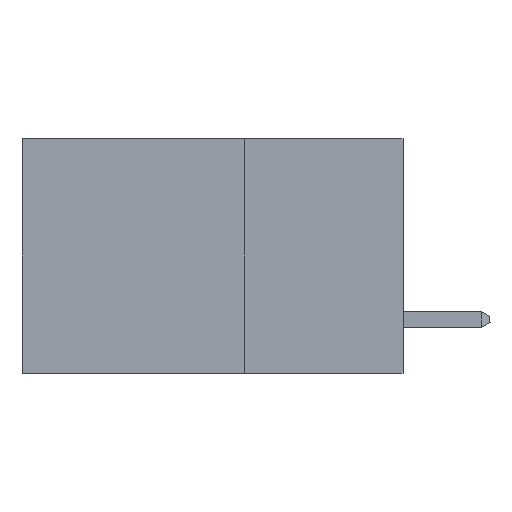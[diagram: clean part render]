
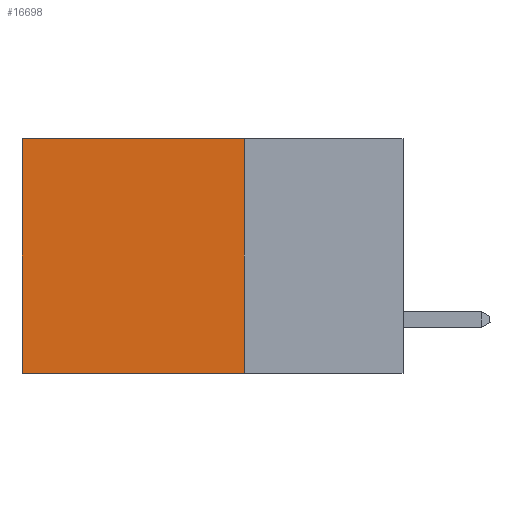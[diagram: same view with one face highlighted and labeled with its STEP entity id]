
A CAD part, left-side view. The second image highlights one B-rep face of the part: STEP entity #16698.
In plain terms, the highlighted planar face has unit normal (-1, 0, 0).
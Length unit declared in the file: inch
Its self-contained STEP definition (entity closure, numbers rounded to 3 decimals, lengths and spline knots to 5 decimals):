
#1212 = EDGE_CURVE ( 'NONE', #16861, #1266, #11007, .T. ) ;
#1266 = VERTEX_POINT ( 'NONE', #9434 ) ;
#1678 = CARTESIAN_POINT ( 'NONE',  ( 0.2875, 0.6, -0.37 ) ) ;
#2645 = DIRECTION ( 'NONE',  ( 0., 0., -1. ) ) ;
#3175 = VECTOR ( 'NONE', #16804, 39.37008 ) ;
#3224 = AXIS2_PLACEMENT_3D ( 'NONE', #14732, #12846, #10677 ) ;
#3611 = FACE_OUTER_BOUND ( 'NONE', #9397, .T. ) ;
#3695 = VERTEX_POINT ( 'NONE', #1678 ) ;
#4485 = ORIENTED_EDGE ( 'NONE', *, *, #14932, .T. ) ;
#5365 = LINE ( 'NONE', #13348, #24353 ) ;
#9069 = CARTESIAN_POINT ( 'NONE',  ( 0.2875, 0.25, 0. ) ) ;
#9397 = EDGE_LOOP ( 'NONE', ( #4485, #13174, #15100, #11902 ) ) ;
#9434 = CARTESIAN_POINT ( 'NONE',  ( 0.2875, 0.25, -0.37 ) ) ;
#10677 = DIRECTION ( 'NONE',  ( 0., 0., -1. ) ) ;
#10802 = EDGE_CURVE ( 'NONE', #16861, #20754, #16137, .T. ) ;
#11007 = LINE ( 'NONE', #9069, #15835 ) ;
#11902 = ORIENTED_EDGE ( 'NONE', *, *, #10802, .T. ) ;
#12846 = DIRECTION ( 'NONE',  ( 1., 0., 0. ) ) ;
#13174 = ORIENTED_EDGE ( 'NONE', *, *, #13213, .F. ) ;
#13213 = EDGE_CURVE ( 'NONE', #1266, #3695, #13503, .T. ) ;
#13348 = CARTESIAN_POINT ( 'NONE',  ( 0.2875, 0.6, 0. ) ) ;
#13503 = LINE ( 'NONE', #16452, #23751 ) ;
#14732 = CARTESIAN_POINT ( 'NONE',  ( 0.2875, 0.25, 0. ) ) ;
#14932 = EDGE_CURVE ( 'NONE', #20754, #3695, #5365, .T. ) ;
#15100 = ORIENTED_EDGE ( 'NONE', *, *, #1212, .F. ) ;
#15835 = VECTOR ( 'NONE', #2645, 39.37008 ) ;
#16137 = LINE ( 'NONE', #24938, #3175 ) ;
#16452 = CARTESIAN_POINT ( 'NONE',  ( 0.2875, 0.25, -0.37 ) ) ;
#16698 = ADVANCED_FACE ( 'NONE', ( #3611 ), #25105, .F. ) ;
#16804 = DIRECTION ( 'NONE',  ( 0., 1., 0. ) ) ;
#16861 = VERTEX_POINT ( 'NONE', #24505 ) ;
#20754 = VERTEX_POINT ( 'NONE', #23098 ) ;
#22325 = DIRECTION ( 'NONE',  ( 0., 1., 0. ) ) ;
#23098 = CARTESIAN_POINT ( 'NONE',  ( 0.2875, 0.6, 0. ) ) ;
#23717 = DIRECTION ( 'NONE',  ( 0., 0., -1. ) ) ;
#23751 = VECTOR ( 'NONE', #22325, 39.37008 ) ;
#24353 = VECTOR ( 'NONE', #23717, 39.37008 ) ;
#24505 = CARTESIAN_POINT ( 'NONE',  ( 0.2875, 0.25, 0. ) ) ;
#24938 = CARTESIAN_POINT ( 'NONE',  ( 0.2875, 0.25, 0. ) ) ;
#25105 = PLANE ( 'NONE',  #3224 ) ;
